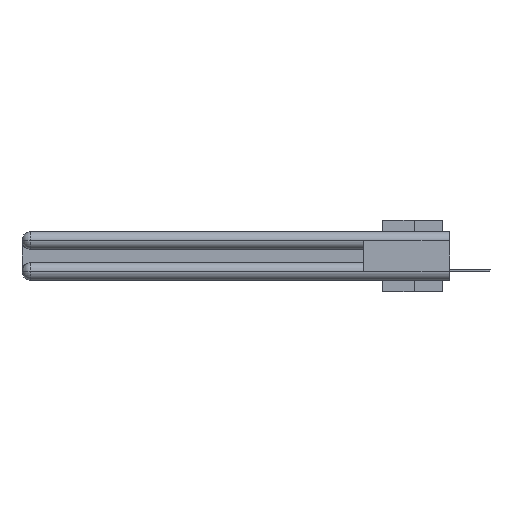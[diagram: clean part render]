
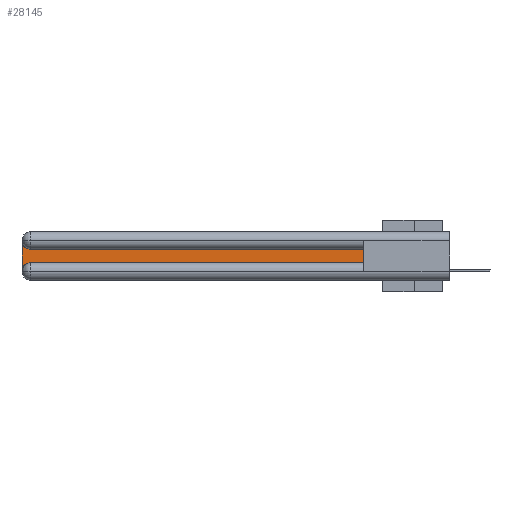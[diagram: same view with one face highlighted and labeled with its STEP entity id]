
A CAD part, left-side view. The second image highlights one B-rep face of the part: STEP entity #28145.
In plain terms, the highlighted planar face has unit normal (-1, 0, 0).
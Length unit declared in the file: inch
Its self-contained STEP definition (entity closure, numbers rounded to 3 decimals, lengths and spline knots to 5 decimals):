
#967 = VECTOR ( 'NONE', #24632, 39.37008 ) ;
#1264 = LINE ( 'NONE', #11605, #967 ) ;
#1615 = LINE ( 'NONE', #19746, #24863 ) ;
#2114 = VERTEX_POINT ( 'NONE', #22537 ) ;
#2382 = DIRECTION ( 'NONE',  ( 0., 0., -1. ) ) ;
#2543 = FACE_OUTER_BOUND ( 'NONE', #30912, .T. ) ;
#4024 = PLANE ( 'NONE',  #28713 ) ;
#4859 = EDGE_CURVE ( 'NONE', #14660, #10670, #32616, .T. ) ;
#6679 = VERTEX_POINT ( 'NONE', #11783 ) ;
#6706 = EDGE_CURVE ( 'NONE', #11053, #2114, #1615, .T. ) ;
#6945 = DIRECTION ( 'NONE',  ( 0., -1., 0. ) ) ;
#8043 = CARTESIAN_POINT ( 'NONE',  ( 0.075, 2.94, -0.1225 ) ) ;
#9062 = DIRECTION ( 'NONE',  ( 0., 0., -1. ) ) ;
#9101 = DIRECTION ( 'NONE',  ( 1., 0., 0. ) ) ;
#9634 = ORIENTED_EDGE ( 'NONE', *, *, #27495, .T. ) ;
#10614 = ORIENTED_EDGE ( 'NONE', *, *, #26622, .T. ) ;
#10670 = VERTEX_POINT ( 'NONE', #18191 ) ;
#11053 = VERTEX_POINT ( 'NONE', #32706 ) ;
#11323 = AXIS2_PLACEMENT_3D ( 'NONE', #27393, #9101, #25186 ) ;
#11394 = VECTOR ( 'NONE', #6945, 39.37008 ) ;
#11605 = CARTESIAN_POINT ( 'NONE',  ( 0.075, 3., -0.2175 ) ) ;
#11783 = CARTESIAN_POINT ( 'NONE',  ( 0.075, 2.94, -0.2175 ) ) ;
#12589 = ORIENTED_EDGE ( 'NONE', *, *, #4859, .T. ) ;
#14529 = CARTESIAN_POINT ( 'NONE',  ( 0.075, 0.6, -0.1225 ) ) ;
#14660 = VERTEX_POINT ( 'NONE', #8043 ) ;
#14670 = CARTESIAN_POINT ( 'NONE',  ( 0.075, 2.94, -0.0625 ) ) ;
#16966 = CARTESIAN_POINT ( 'NONE',  ( 0.075, 0.6, -0.2175 ) ) ;
#17078 = LINE ( 'NONE', #14529, #18765 ) ;
#17490 = ORIENTED_EDGE ( 'NONE', *, *, #6706, .T. ) ;
#17852 = CIRCLE ( 'NONE', #11323, 0.06 ) ;
#18184 = DIRECTION ( 'NONE',  ( 0., 0., 1. ) ) ;
#18191 = CARTESIAN_POINT ( 'NONE',  ( 0.075, 3., -0.0625 ) ) ;
#18765 = VECTOR ( 'NONE', #18920, 39.37008 ) ;
#18920 = DIRECTION ( 'NONE',  ( 0., 1., 0. ) ) ;
#19484 = LINE ( 'NONE', #16966, #11394 ) ;
#19746 = CARTESIAN_POINT ( 'NONE',  ( 0.075, 0.6, -0.2175 ) ) ;
#20506 = DIRECTION ( 'NONE',  ( 1., 0., 0. ) ) ;
#21840 = EDGE_CURVE ( 'NONE', #2114, #14660, #17078, .T. ) ;
#22537 = CARTESIAN_POINT ( 'NONE',  ( 0.075, 0.6, -0.1225 ) ) ;
#23493 = EDGE_CURVE ( 'NONE', #10670, #28348, #1264, .T. ) ;
#23698 = CARTESIAN_POINT ( 'NONE',  ( 0.075, 3., -0.1225 ) ) ;
#23707 = ORIENTED_EDGE ( 'NONE', *, *, #21840, .T. ) ;
#24632 = DIRECTION ( 'NONE',  ( 0., 0., -1. ) ) ;
#24863 = VECTOR ( 'NONE', #18184, 39.37008 ) ;
#25186 = DIRECTION ( 'NONE',  ( 0., 0., -1. ) ) ;
#26407 = CARTESIAN_POINT ( 'NONE',  ( 0.075, 3., -0.2775 ) ) ;
#26622 = EDGE_CURVE ( 'NONE', #28348, #6679, #17852, .T. ) ;
#26673 = AXIS2_PLACEMENT_3D ( 'NONE', #14670, #32766, #9062 ) ;
#27393 = CARTESIAN_POINT ( 'NONE',  ( 0.075, 2.94, -0.2775 ) ) ;
#27495 = EDGE_CURVE ( 'NONE', #6679, #11053, #19484, .T. ) ;
#28145 = ADVANCED_FACE ( 'NONE', ( #2543 ), #4024, .F. ) ;
#28348 = VERTEX_POINT ( 'NONE', #26407 ) ;
#28713 = AXIS2_PLACEMENT_3D ( 'NONE', #23698, #20506, #2382 ) ;
#30912 = EDGE_LOOP ( 'NONE', ( #23707, #12589, #32681, #10614, #9634, #17490 ) ) ;
#32616 = CIRCLE ( 'NONE', #26673, 0.06 ) ;
#32681 = ORIENTED_EDGE ( 'NONE', *, *, #23493, .T. ) ;
#32706 = CARTESIAN_POINT ( 'NONE',  ( 0.075, 0.6, -0.2175 ) ) ;
#32766 = DIRECTION ( 'NONE',  ( 1., 0., 0. ) ) ;
